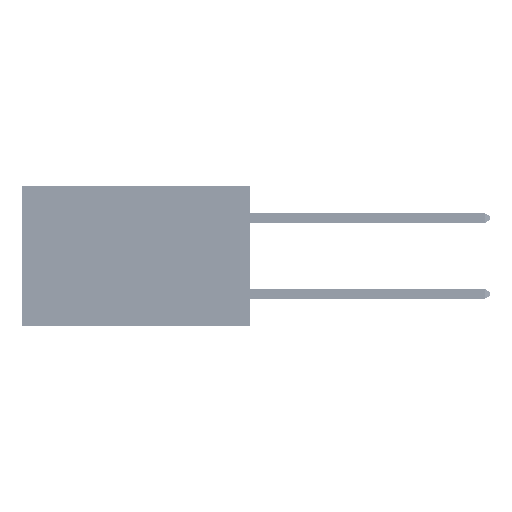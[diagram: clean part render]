
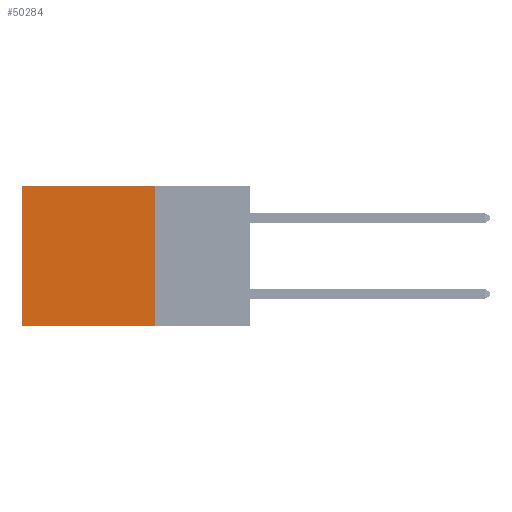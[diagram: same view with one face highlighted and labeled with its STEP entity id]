
A CAD part, left-side view. The second image highlights one B-rep face of the part: STEP entity #50284.
In plain terms, the highlighted planar face has unit normal (-1, 0, 0).
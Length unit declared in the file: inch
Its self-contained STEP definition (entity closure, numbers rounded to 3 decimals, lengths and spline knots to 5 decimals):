
#254 = VECTOR ( 'NONE', #3549, 39.37008 ) ;
#2231 = LINE ( 'NONE', #18591, #25750 ) ;
#3549 = DIRECTION ( 'NONE',  ( 0., 0., -1. ) ) ;
#5031 = DIRECTION ( 'NONE',  ( 0., 0., -1. ) ) ;
#5652 = CARTESIAN_POINT ( 'NONE',  ( 0.2875, 0.25, 0. ) ) ;
#6016 = FACE_OUTER_BOUND ( 'NONE', #21172, .T. ) ;
#6749 = ORIENTED_EDGE ( 'NONE', *, *, #49856, .F. ) ;
#9063 = LINE ( 'NONE', #25416, #39488 ) ;
#11868 = VERTEX_POINT ( 'NONE', #21933 ) ;
#13949 = DIRECTION ( 'NONE',  ( 0., 1., 0. ) ) ;
#14637 = EDGE_CURVE ( 'NONE', #20770, #11868, #2231, .T. ) ;
#18591 = CARTESIAN_POINT ( 'NONE',  ( 0.2875, 0.25, 0. ) ) ;
#18642 = CARTESIAN_POINT ( 'NONE',  ( 0.2875, 0.25, -0.37 ) ) ;
#19859 = EDGE_CURVE ( 'NONE', #11868, #47001, #9063, .T. ) ;
#20770 = VERTEX_POINT ( 'NONE', #5652 ) ;
#21172 = EDGE_LOOP ( 'NONE', ( #31243, #6749, #45767, #36853 ) ) ;
#21933 = CARTESIAN_POINT ( 'NONE',  ( 0.2875, 0.6, 0. ) ) ;
#24205 = CARTESIAN_POINT ( 'NONE',  ( 0.2875, 0.25, 0. ) ) ;
#25416 = CARTESIAN_POINT ( 'NONE',  ( 0.2875, 0.6, 0. ) ) ;
#25750 = VECTOR ( 'NONE', #26108, 39.37008 ) ;
#26108 = DIRECTION ( 'NONE',  ( 0., 1., 0. ) ) ;
#26146 = PLANE ( 'NONE',  #49261 ) ;
#27274 = VERTEX_POINT ( 'NONE', #18642 ) ;
#29061 = EDGE_CURVE ( 'NONE', #20770, #27274, #48834, .T. ) ;
#29514 = CARTESIAN_POINT ( 'NONE',  ( 0.2875, 0.6, -0.37 ) ) ;
#31243 = ORIENTED_EDGE ( 'NONE', *, *, #19859, .T. ) ;
#36853 = ORIENTED_EDGE ( 'NONE', *, *, #14637, .T. ) ;
#38729 = DIRECTION ( 'NONE',  ( 0., 0., -1. ) ) ;
#39488 = VECTOR ( 'NONE', #5031, 39.37008 ) ;
#43034 = DIRECTION ( 'NONE',  ( 1., 0., 0. ) ) ;
#43295 = CARTESIAN_POINT ( 'NONE',  ( 0.2875, 0.25, 0. ) ) ;
#44131 = VECTOR ( 'NONE', #13949, 39.37008 ) ;
#45767 = ORIENTED_EDGE ( 'NONE', *, *, #29061, .F. ) ;
#47001 = VERTEX_POINT ( 'NONE', #29514 ) ;
#48834 = LINE ( 'NONE', #24205, #254 ) ;
#49261 = AXIS2_PLACEMENT_3D ( 'NONE', #43295, #43034, #38729 ) ;
#49856 = EDGE_CURVE ( 'NONE', #27274, #47001, #50132, .T. ) ;
#50132 = LINE ( 'NONE', #51649, #44131 ) ;
#50284 = ADVANCED_FACE ( 'NONE', ( #6016 ), #26146, .F. ) ;
#51649 = CARTESIAN_POINT ( 'NONE',  ( 0.2875, 0.25, -0.37 ) ) ;
